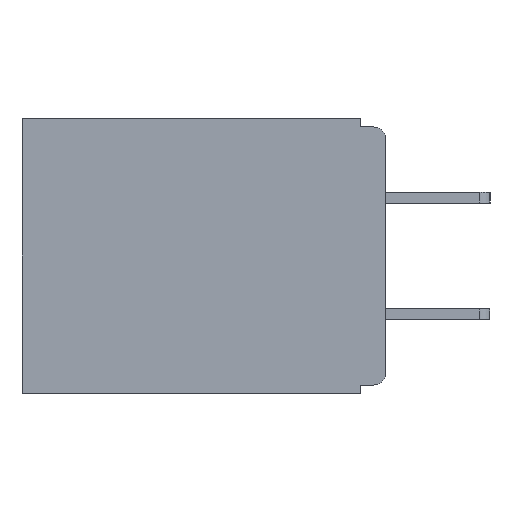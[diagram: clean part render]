
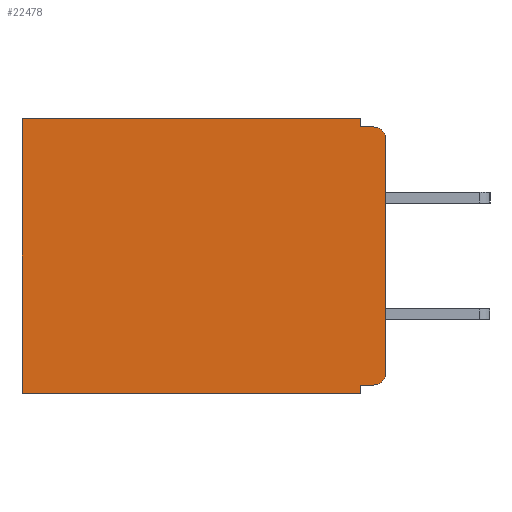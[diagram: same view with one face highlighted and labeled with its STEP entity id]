
A CAD part, left-side view. The second image highlights one B-rep face of the part: STEP entity #22478.
In plain terms, the highlighted planar face has unit normal (-1, 0, 0).
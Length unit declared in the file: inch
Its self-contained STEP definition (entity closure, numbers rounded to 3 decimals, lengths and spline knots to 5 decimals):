
#9 = CARTESIAN_POINT ( 'NONE',  ( 0.3, 0., -0.33 ) ) ;
#40 = VERTEX_POINT ( 'NONE', #14820 ) ;
#447 = CARTESIAN_POINT ( 'NONE',  ( 0.3, 0., -0.01 ) ) ;
#881 = CIRCLE ( 'NONE', #6727, 0.015 ) ;
#947 = EDGE_CURVE ( 'NONE', #12801, #21290, #14193, .T. ) ;
#1056 = DIRECTION ( 'NONE',  ( -1., 0., 0. ) ) ;
#1810 = DIRECTION ( 'NONE',  ( 1., 0., 0. ) ) ;
#2038 = CARTESIAN_POINT ( 'NONE',  ( 0.3, 0.437, 0. ) ) ;
#2116 = ORIENTED_EDGE ( 'NONE', *, *, #947, .F. ) ;
#2791 = CARTESIAN_POINT ( 'NONE',  ( 0.3, 0.015, -0.025 ) ) ;
#3049 = EDGE_CURVE ( 'NONE', #12801, #14084, #21370, .T. ) ;
#3327 = VECTOR ( 'NONE', #17410, 39.37008 ) ;
#3570 = CARTESIAN_POINT ( 'NONE',  ( 0.3, 0.031, -0.33 ) ) ;
#3791 = EDGE_CURVE ( 'NONE', #40, #9442, #881, .T. ) ;
#3819 = EDGE_CURVE ( 'NONE', #21290, #9442, #4526, .T. ) ;
#4261 = CARTESIAN_POINT ( 'NONE',  ( 0.3, 0.031, -0.32 ) ) ;
#4351 = VERTEX_POINT ( 'NONE', #3570 ) ;
#4365 = DIRECTION ( 'NONE',  ( -1., 0., 0. ) ) ;
#4526 = LINE ( 'NONE', #447, #18440 ) ;
#5464 = VERTEX_POINT ( 'NONE', #7028 ) ;
#5940 = LINE ( 'NONE', #22421, #6502 ) ;
#5966 = CARTESIAN_POINT ( 'NONE',  ( 0.3, 0., -0.305 ) ) ;
#6400 = DIRECTION ( 'NONE',  ( 0., -1., 0. ) ) ;
#6419 = VERTEX_POINT ( 'NONE', #5966 ) ;
#6502 = VECTOR ( 'NONE', #12135, 39.37008 ) ;
#6727 = AXIS2_PLACEMENT_3D ( 'NONE', #2791, #4365, #20323 ) ;
#6982 = EDGE_CURVE ( 'NONE', #4351, #7790, #17726, .T. ) ;
#7028 = CARTESIAN_POINT ( 'NONE',  ( 0.3, 0.015, -0.32 ) ) ;
#7105 = CARTESIAN_POINT ( 'NONE',  ( 0.3, 0.031, 0. ) ) ;
#7628 = DIRECTION ( 'NONE',  ( 0., 1., 0. ) ) ;
#7634 = CARTESIAN_POINT ( 'NONE',  ( 0.3, 0., 0. ) ) ;
#7689 = ORIENTED_EDGE ( 'NONE', *, *, #3049, .T. ) ;
#7790 = VERTEX_POINT ( 'NONE', #8039 ) ;
#8039 = CARTESIAN_POINT ( 'NONE',  ( 0.3, 0.437, -0.33 ) ) ;
#8041 = LINE ( 'NONE', #22444, #3327 ) ;
#8700 = CARTESIAN_POINT ( 'NONE',  ( 0.3, 0.031, -0.01 ) ) ;
#9046 = ORIENTED_EDGE ( 'NONE', *, *, #11335, .T. ) ;
#9089 = VECTOR ( 'NONE', #14044, 39.37008 ) ;
#9131 = ORIENTED_EDGE ( 'NONE', *, *, #3819, .F. ) ;
#9246 = EDGE_CURVE ( 'NONE', #5464, #15197, #12744, .T. ) ;
#9442 = VERTEX_POINT ( 'NONE', #11820 ) ;
#9919 = AXIS2_PLACEMENT_3D ( 'NONE', #9, #1810, #14059 ) ;
#10013 = LINE ( 'NONE', #20847, #19240 ) ;
#10221 = EDGE_CURVE ( 'NONE', #40, #6419, #10013, .T. ) ;
#10260 = EDGE_LOOP ( 'NONE', ( #11831, #17539, #9131, #2116, #7689, #9046, #11414, #12772, #13570, #13523 ) ) ;
#10592 = PLANE ( 'NONE',  #9919 ) ;
#11335 = EDGE_CURVE ( 'NONE', #14084, #7790, #5940, .T. ) ;
#11414 = ORIENTED_EDGE ( 'NONE', *, *, #6982, .F. ) ;
#11600 = CARTESIAN_POINT ( 'NONE',  ( 0.3, 0.015, -0.305 ) ) ;
#11820 = CARTESIAN_POINT ( 'NONE',  ( 0.3, 0.015, -0.01 ) ) ;
#11831 = ORIENTED_EDGE ( 'NONE', *, *, #10221, .F. ) ;
#12135 = DIRECTION ( 'NONE',  ( 0., 0., -1. ) ) ;
#12252 = DIRECTION ( 'NONE',  ( 0., 0., -1. ) ) ;
#12350 = AXIS2_PLACEMENT_3D ( 'NONE', #11600, #1056, #13644 ) ;
#12489 = DIRECTION ( 'NONE',  ( 0., 1., 0. ) ) ;
#12599 = FACE_OUTER_BOUND ( 'NONE', #10260, .T. ) ;
#12733 = EDGE_CURVE ( 'NONE', #15197, #4351, #8041, .T. ) ;
#12744 = LINE ( 'NONE', #15711, #21367 ) ;
#12772 = ORIENTED_EDGE ( 'NONE', *, *, #12733, .F. ) ;
#12801 = VERTEX_POINT ( 'NONE', #20965 ) ;
#13077 = VECTOR ( 'NONE', #7628, 39.37008 ) ;
#13523 = ORIENTED_EDGE ( 'NONE', *, *, #21690, .T. ) ;
#13570 = ORIENTED_EDGE ( 'NONE', *, *, #9246, .F. ) ;
#13644 = DIRECTION ( 'NONE',  ( 0., 0., -1. ) ) ;
#14044 = DIRECTION ( 'NONE',  ( 0., 0., -1. ) ) ;
#14059 = DIRECTION ( 'NONE',  ( 0., 0., -1. ) ) ;
#14084 = VERTEX_POINT ( 'NONE', #2038 ) ;
#14193 = LINE ( 'NONE', #7105, #9089 ) ;
#14820 = CARTESIAN_POINT ( 'NONE',  ( 0.3, 0., -0.025 ) ) ;
#15197 = VERTEX_POINT ( 'NONE', #4261 ) ;
#15711 = CARTESIAN_POINT ( 'NONE',  ( 0.3, 0., -0.32 ) ) ;
#15750 = VECTOR ( 'NONE', #12489, 39.37008 ) ;
#16204 = CIRCLE ( 'NONE', #12350, 0.015 ) ;
#16271 = CARTESIAN_POINT ( 'NONE',  ( 0.3, 0., -0.33 ) ) ;
#17410 = DIRECTION ( 'NONE',  ( 0., 0., -1. ) ) ;
#17539 = ORIENTED_EDGE ( 'NONE', *, *, #3791, .T. ) ;
#17726 = LINE ( 'NONE', #16271, #13077 ) ;
#18440 = VECTOR ( 'NONE', #6400, 39.37008 ) ;
#19240 = VECTOR ( 'NONE', #12252, 39.37008 ) ;
#20323 = DIRECTION ( 'NONE',  ( 0., 0., -1. ) ) ;
#20807 = DIRECTION ( 'NONE',  ( 0., 1., 0. ) ) ;
#20847 = CARTESIAN_POINT ( 'NONE',  ( 0.3, 0., -0.33 ) ) ;
#20965 = CARTESIAN_POINT ( 'NONE',  ( 0.3, 0.031, 0. ) ) ;
#21290 = VERTEX_POINT ( 'NONE', #8700 ) ;
#21367 = VECTOR ( 'NONE', #20807, 39.37008 ) ;
#21370 = LINE ( 'NONE', #7634, #15750 ) ;
#21690 = EDGE_CURVE ( 'NONE', #5464, #6419, #16204, .T. ) ;
#22421 = CARTESIAN_POINT ( 'NONE',  ( 0.3, 0.437, -0.33 ) ) ;
#22444 = CARTESIAN_POINT ( 'NONE',  ( 0.3, 0.031, -0.33 ) ) ;
#22478 = ADVANCED_FACE ( 'NONE', ( #12599 ), #10592, .F. ) ;
